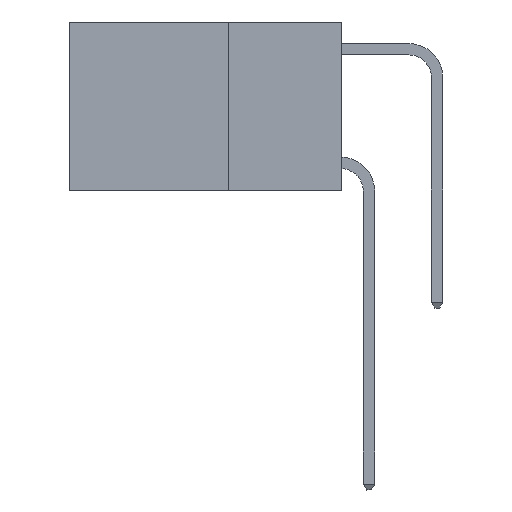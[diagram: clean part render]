
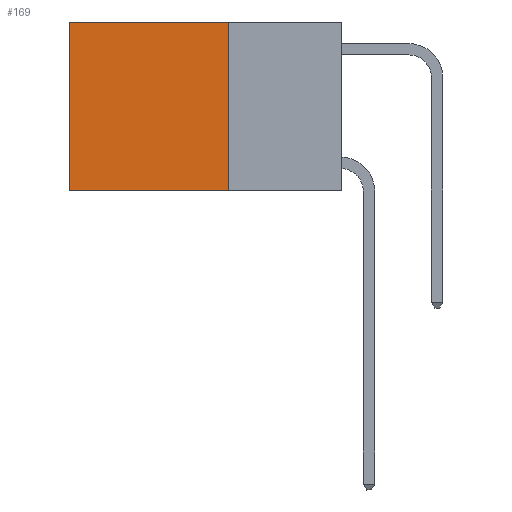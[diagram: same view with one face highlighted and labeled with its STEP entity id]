
A CAD part, left-side view. The second image highlights one B-rep face of the part: STEP entity #169.
In plain terms, the highlighted planar face has unit normal (-1, 0, 0).
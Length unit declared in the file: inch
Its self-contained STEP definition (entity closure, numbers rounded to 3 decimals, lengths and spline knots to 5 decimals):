
#42 = VECTOR ( 'NONE', #8677, 39.37008 ) ;
#169 = ADVANCED_FACE ( 'NONE', ( #1179 ), #15710, .F. ) ;
#517 = VERTEX_POINT ( 'NONE', #6568 ) ;
#521 = VERTEX_POINT ( 'NONE', #17101 ) ;
#1179 = FACE_OUTER_BOUND ( 'NONE', #2600, .T. ) ;
#1737 = CARTESIAN_POINT ( 'NONE',  ( 0.2625, 0.25, -0.37 ) ) ;
#1760 = CARTESIAN_POINT ( 'NONE',  ( 0.2625, 0.6, -0.37 ) ) ;
#2151 = VERTEX_POINT ( 'NONE', #1760 ) ;
#2274 = CARTESIAN_POINT ( 'NONE',  ( 0.2625, 0.25, 0. ) ) ;
#2600 = EDGE_LOOP ( 'NONE', ( #6873, #4811, #19031, #9141 ) ) ;
#4495 = VERTEX_POINT ( 'NONE', #21038 ) ;
#4811 = ORIENTED_EDGE ( 'NONE', *, *, #18839, .F. ) ;
#5274 = DIRECTION ( 'NONE',  ( 0., 0., -1. ) ) ;
#6568 = CARTESIAN_POINT ( 'NONE',  ( 0.2625, 0.25, -0.37 ) ) ;
#6873 = ORIENTED_EDGE ( 'NONE', *, *, #23143, .T. ) ;
#7433 = EDGE_CURVE ( 'NONE', #4495, #517, #11992, .T. ) ;
#7792 = VECTOR ( 'NONE', #10355, 39.37008 ) ;
#8298 = VECTOR ( 'NONE', #9426, 39.37008 ) ;
#8372 = CARTESIAN_POINT ( 'NONE',  ( 0.2625, 0.25, 0. ) ) ;
#8677 = DIRECTION ( 'NONE',  ( 0., 1., 0. ) ) ;
#9141 = ORIENTED_EDGE ( 'NONE', *, *, #19427, .T. ) ;
#9426 = DIRECTION ( 'NONE',  ( 0., 1., 0. ) ) ;
#10355 = DIRECTION ( 'NONE',  ( 0., 0., -1. ) ) ;
#11227 = AXIS2_PLACEMENT_3D ( 'NONE', #8372, #20774, #13974 ) ;
#11992 = LINE ( 'NONE', #13752, #7792 ) ;
#13752 = CARTESIAN_POINT ( 'NONE',  ( 0.2625, 0.25, 0. ) ) ;
#13974 = DIRECTION ( 'NONE',  ( 0., 0., -1. ) ) ;
#14017 = VECTOR ( 'NONE', #5274, 39.37008 ) ;
#14146 = LINE ( 'NONE', #17662, #14017 ) ;
#15149 = LINE ( 'NONE', #2274, #8298 ) ;
#15710 = PLANE ( 'NONE',  #11227 ) ;
#17101 = CARTESIAN_POINT ( 'NONE',  ( 0.2625, 0.6, 0. ) ) ;
#17662 = CARTESIAN_POINT ( 'NONE',  ( 0.2625, 0.6, 0. ) ) ;
#17804 = LINE ( 'NONE', #1737, #42 ) ;
#18839 = EDGE_CURVE ( 'NONE', #517, #2151, #17804, .T. ) ;
#19031 = ORIENTED_EDGE ( 'NONE', *, *, #7433, .F. ) ;
#19427 = EDGE_CURVE ( 'NONE', #4495, #521, #15149, .T. ) ;
#20774 = DIRECTION ( 'NONE',  ( 1., 0., 0. ) ) ;
#21038 = CARTESIAN_POINT ( 'NONE',  ( 0.2625, 0.25, 0. ) ) ;
#23143 = EDGE_CURVE ( 'NONE', #521, #2151, #14146, .T. ) ;
